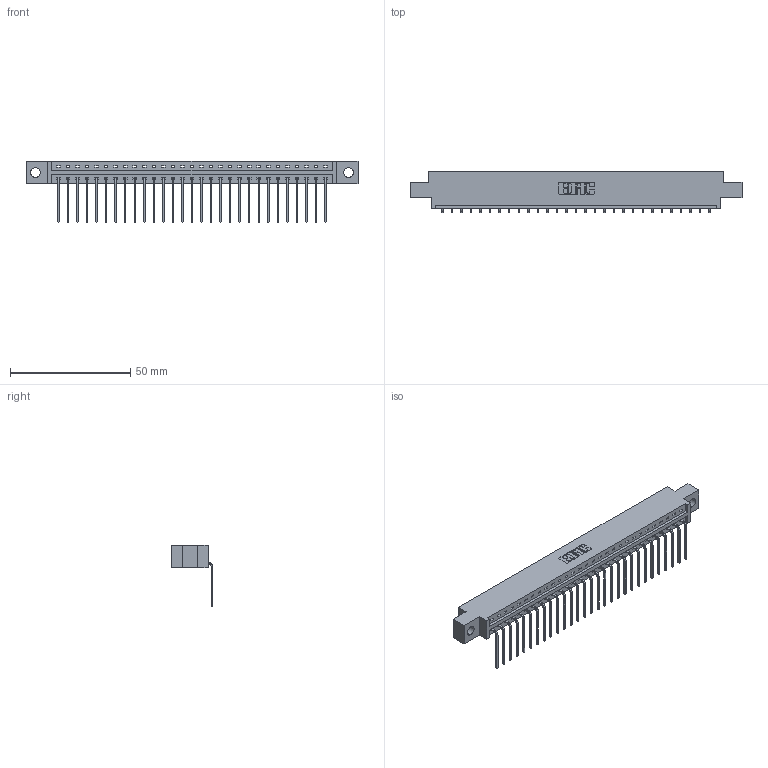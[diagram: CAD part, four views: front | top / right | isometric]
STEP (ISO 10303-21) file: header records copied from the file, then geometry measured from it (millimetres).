
FILE_DESCRIPTION (( 'STEP AP203' ), '1' );
FILE_NAME ('337-029-559-604.STEP', '2019-09-30T22:59:28', ( '' ), ( '' ), 'SwSTEP 2.0', 'SolidWorks 2016', '' );
FILE_SCHEMA (( 'CONFIG_CONTROL_DESIGN' ));
Length unit declared in the file: inch
Products named in the file (3): 337-029-559-604; 345-292-001_558 559 Tail - 1; 337 Part_0.170 Offset - 0.156 Dia-TH
Assembly tree (30 placements, depth 2):
  337-029-559-604
    337 Part_0.170 Offset - 0.156 Dia-TH
    345-292-001_558 559 Tail - 1  x29
Bounding box: 137.92 x 17.09 x 25.53 mm (x, y, z)
Volume: 14063.3 mm3; surface area: 14945.4 mm2
Topology: 30 solids, 30 shells, 1974 faces, 5949 edges, 3926 vertices
Faces by surface type: plane 1466, cylinder 508
Entity records: 23457 total; most frequent: CARTESIAN_POINT 4093, ORIENTED_EDGE 4058, DIRECTION 3471, EDGE_CURVE 2029, VECTOR 1901, LINE 1901, VERTEX_POINT 1350, AXIS2_PLACEMENT_3D 785
